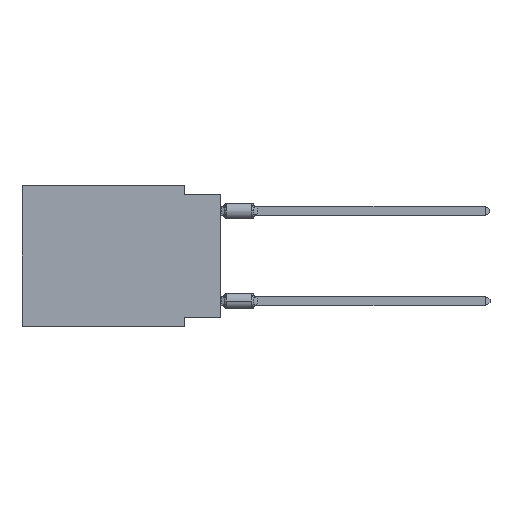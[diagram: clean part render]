
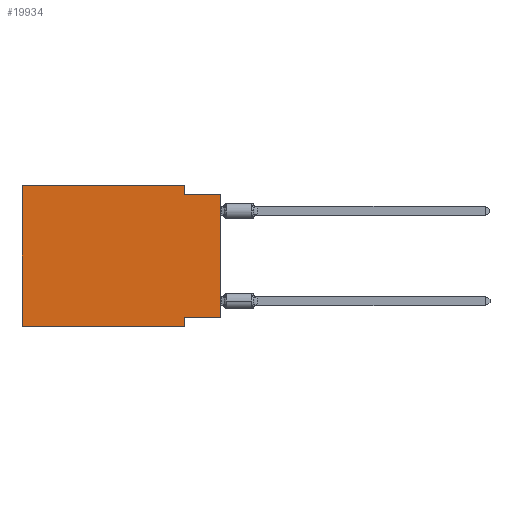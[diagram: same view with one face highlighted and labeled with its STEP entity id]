
A CAD part, left-side view. The second image highlights one B-rep face of the part: STEP entity #19934.
In plain terms, the highlighted planar face has unit normal (-1, 0, 0).
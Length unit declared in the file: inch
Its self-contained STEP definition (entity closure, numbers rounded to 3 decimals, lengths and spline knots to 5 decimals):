
#863 = CARTESIAN_POINT ( 'NONE',  ( 0., 0.55, -0.39 ) ) ;
#1164 = VERTEX_POINT ( 'NONE', #59467 ) ;
#2396 = VERTEX_POINT ( 'NONE', #37139 ) ;
#3654 = VECTOR ( 'NONE', #18641, 39.37008 ) ;
#4626 = LINE ( 'NONE', #46952, #53229 ) ;
#5168 = DIRECTION ( 'NONE',  ( 0., -1., 0. ) ) ;
#6112 = VERTEX_POINT ( 'NONE', #39048 ) ;
#7760 = EDGE_CURVE ( 'NONE', #8686, #46636, #15499, .T. ) ;
#8335 = ORIENTED_EDGE ( 'NONE', *, *, #7760, .T. ) ;
#8686 = VERTEX_POINT ( 'NONE', #863 ) ;
#9267 = CARTESIAN_POINT ( 'NONE',  ( 0., 0.55, 0. ) ) ;
#9583 = VECTOR ( 'NONE', #21768, 39.37008 ) ;
#10352 = PLANE ( 'NONE',  #29716 ) ;
#10369 = EDGE_CURVE ( 'NONE', #6112, #2396, #12360, .T. ) ;
#12360 = LINE ( 'NONE', #45613, #9583 ) ;
#12902 = EDGE_CURVE ( 'NONE', #49336, #6112, #19102, .T. ) ;
#13623 = CARTESIAN_POINT ( 'NONE',  ( 0., 0., -0.365 ) ) ;
#14398 = CARTESIAN_POINT ( 'NONE',  ( 0., 0.1, 0. ) ) ;
#15499 = LINE ( 'NONE', #38104, #35559 ) ;
#18015 = LINE ( 'NONE', #13623, #3654 ) ;
#18641 = DIRECTION ( 'NONE',  ( 0., 1., 0. ) ) ;
#18817 = EDGE_LOOP ( 'NONE', ( #40207, #55085, #60985, #55993, #43993, #8335, #48042, #30496 ) ) ;
#18992 = LINE ( 'NONE', #9267, #42612 ) ;
#19102 = LINE ( 'NONE', #14398, #35833 ) ;
#19770 = DIRECTION ( 'NONE',  ( 1., 0., 0. ) ) ;
#19934 = ADVANCED_FACE ( 'NONE', ( #20703 ), #10352, .F. ) ;
#20703 = FACE_OUTER_BOUND ( 'NONE', #18817, .T. ) ;
#21768 = DIRECTION ( 'NONE',  ( 0., -1., 0. ) ) ;
#21881 = CARTESIAN_POINT ( 'NONE',  ( 0., 0.1, -0.39 ) ) ;
#23516 = VECTOR ( 'NONE', #23725, 39.37008 ) ;
#23725 = DIRECTION ( 'NONE',  ( 0., 0., 1. ) ) ;
#26926 = LINE ( 'NONE', #45753, #45493 ) ;
#29716 = AXIS2_PLACEMENT_3D ( 'NONE', #48014, #19770, #43910 ) ;
#29778 = DIRECTION ( 'NONE',  ( 0., 0., -1. ) ) ;
#30496 = ORIENTED_EDGE ( 'NONE', *, *, #58407, .F. ) ;
#32181 = CARTESIAN_POINT ( 'NONE',  ( 0., 0., 0. ) ) ;
#33232 = EDGE_CURVE ( 'NONE', #46976, #49336, #26926, .T. ) ;
#33746 = DIRECTION ( 'NONE',  ( 0., 0., 1. ) ) ;
#35559 = VECTOR ( 'NONE', #5168, 39.37008 ) ;
#35833 = VECTOR ( 'NONE', #29778, 39.37008 ) ;
#37139 = CARTESIAN_POINT ( 'NONE',  ( 0., 0., -0.025 ) ) ;
#38104 = CARTESIAN_POINT ( 'NONE',  ( 0., 0.55, -0.39 ) ) ;
#38584 = EDGE_CURVE ( 'NONE', #8686, #46976, #18992, .T. ) ;
#39048 = CARTESIAN_POINT ( 'NONE',  ( 0., 0.1, -0.025 ) ) ;
#40207 = ORIENTED_EDGE ( 'NONE', *, *, #56727, .T. ) ;
#40408 = CARTESIAN_POINT ( 'NONE',  ( 0., 0.1, -0.365 ) ) ;
#42549 = DIRECTION ( 'NONE',  ( 0., 0., -1. ) ) ;
#42612 = VECTOR ( 'NONE', #33746, 39.37008 ) ;
#43910 = DIRECTION ( 'NONE',  ( 0., 0., -1. ) ) ;
#43993 = ORIENTED_EDGE ( 'NONE', *, *, #38584, .F. ) ;
#45493 = VECTOR ( 'NONE', #46048, 39.37008 ) ;
#45613 = CARTESIAN_POINT ( 'NONE',  ( 0., 0., -0.025 ) ) ;
#45753 = CARTESIAN_POINT ( 'NONE',  ( 0., 0.55, 0. ) ) ;
#46048 = DIRECTION ( 'NONE',  ( 0., -1., 0. ) ) ;
#46636 = VERTEX_POINT ( 'NONE', #21881 ) ;
#46952 = CARTESIAN_POINT ( 'NONE',  ( 0., 0.1, -0.39 ) ) ;
#46976 = VERTEX_POINT ( 'NONE', #58339 ) ;
#47246 = EDGE_CURVE ( 'NONE', #48474, #46636, #4626, .T. ) ;
#48014 = CARTESIAN_POINT ( 'NONE',  ( 0., 0.55, 0. ) ) ;
#48042 = ORIENTED_EDGE ( 'NONE', *, *, #47246, .F. ) ;
#48474 = VERTEX_POINT ( 'NONE', #40408 ) ;
#49336 = VERTEX_POINT ( 'NONE', #57735 ) ;
#53229 = VECTOR ( 'NONE', #42549, 39.37008 ) ;
#55085 = ORIENTED_EDGE ( 'NONE', *, *, #10369, .F. ) ;
#55993 = ORIENTED_EDGE ( 'NONE', *, *, #33232, .F. ) ;
#56361 = LINE ( 'NONE', #32181, #23516 ) ;
#56727 = EDGE_CURVE ( 'NONE', #1164, #2396, #56361, .T. ) ;
#57735 = CARTESIAN_POINT ( 'NONE',  ( 0., 0.1, 0. ) ) ;
#58339 = CARTESIAN_POINT ( 'NONE',  ( 0., 0.55, 0. ) ) ;
#58407 = EDGE_CURVE ( 'NONE', #1164, #48474, #18015, .T. ) ;
#59467 = CARTESIAN_POINT ( 'NONE',  ( 0., 0., -0.365 ) ) ;
#60985 = ORIENTED_EDGE ( 'NONE', *, *, #12902, .F. ) ;
